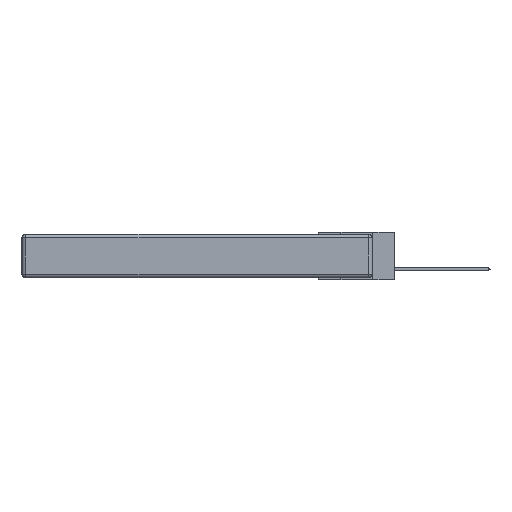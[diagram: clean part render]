
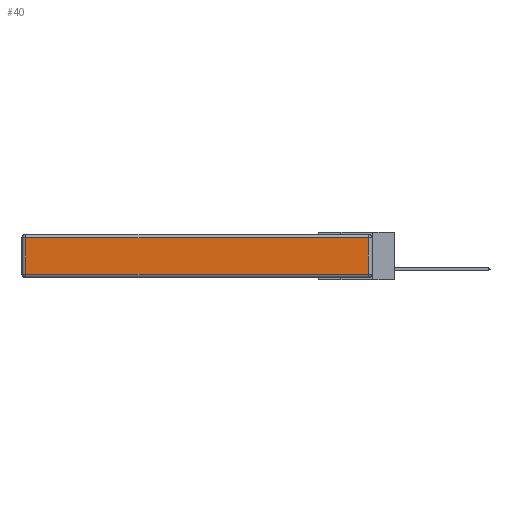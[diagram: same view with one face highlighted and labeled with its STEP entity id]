
A CAD part, left-side view. The second image highlights one B-rep face of the part: STEP entity #40.
In plain terms, the highlighted planar face has unit normal (-1, 0, 0).
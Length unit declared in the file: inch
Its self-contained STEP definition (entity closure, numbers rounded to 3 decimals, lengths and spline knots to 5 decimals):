
#40 = ADVANCED_FACE ( 'NONE', ( #24130 ), #11914, .T. ) ;
#485 = LINE ( 'NONE', #15157, #26127 ) ;
#1071 = EDGE_CURVE ( 'NONE', #5950, #18818, #15418, .T. ) ;
#2519 = ORIENTED_EDGE ( 'NONE', *, *, #5761, .T. ) ;
#3754 = DIRECTION ( 'NONE',  ( -1., 0., 0. ) ) ;
#3831 = VECTOR ( 'NONE', #7269, 39.37008 ) ;
#4460 = DIRECTION ( 'NONE',  ( 0., 0., -1. ) ) ;
#4803 = LINE ( 'NONE', #22928, #15100 ) ;
#5084 = CARTESIAN_POINT ( 'NONE',  ( 0., 2.72, -0.313 ) ) ;
#5466 = CARTESIAN_POINT ( 'NONE',  ( 0., 0.03, -0.343 ) ) ;
#5761 = EDGE_CURVE ( 'NONE', #18818, #6465, #485, .T. ) ;
#5910 = DIRECTION ( 'NONE',  ( 0., 0., 1. ) ) ;
#5950 = VERTEX_POINT ( 'NONE', #21276 ) ;
#6465 = VERTEX_POINT ( 'NONE', #13262 ) ;
#7269 = DIRECTION ( 'NONE',  ( 0., 0., 1. ) ) ;
#8043 = CARTESIAN_POINT ( 'NONE',  ( 0., 0., -0.343 ) ) ;
#11120 = EDGE_CURVE ( 'NONE', #17158, #5950, #4803, .T. ) ;
#11696 = ORIENTED_EDGE ( 'NONE', *, *, #11120, .T. ) ;
#11914 = PLANE ( 'NONE',  #11932 ) ;
#11932 = AXIS2_PLACEMENT_3D ( 'NONE', #8043, #3754, #5910 ) ;
#12120 = ORIENTED_EDGE ( 'NONE', *, *, #1071, .T. ) ;
#12388 = VECTOR ( 'NONE', #4460, 39.37008 ) ;
#12735 = EDGE_CURVE ( 'NONE', #6465, #17158, #19508, .T. ) ;
#13262 = CARTESIAN_POINT ( 'NONE',  ( 0., 2.72, -0.03 ) ) ;
#14337 = DIRECTION ( 'NONE',  ( 0., -1., 0. ) ) ;
#14644 = CARTESIAN_POINT ( 'NONE',  ( 0., 2.72, -0.343 ) ) ;
#15100 = VECTOR ( 'NONE', #14337, 39.37008 ) ;
#15157 = CARTESIAN_POINT ( 'NONE',  ( 0., 2.75, -0.03 ) ) ;
#15418 = LINE ( 'NONE', #5466, #3831 ) ;
#16150 = ORIENTED_EDGE ( 'NONE', *, *, #12735, .T. ) ;
#16777 = CARTESIAN_POINT ( 'NONE',  ( 0., 0.03, -0.03 ) ) ;
#17158 = VERTEX_POINT ( 'NONE', #5084 ) ;
#18818 = VERTEX_POINT ( 'NONE', #16777 ) ;
#19508 = LINE ( 'NONE', #14644, #12388 ) ;
#21191 = DIRECTION ( 'NONE',  ( 0., 1., 0. ) ) ;
#21276 = CARTESIAN_POINT ( 'NONE',  ( 0., 0.03, -0.313 ) ) ;
#22928 = CARTESIAN_POINT ( 'NONE',  ( 0., 0., -0.313 ) ) ;
#24130 = FACE_OUTER_BOUND ( 'NONE', #24866, .T. ) ;
#24866 = EDGE_LOOP ( 'NONE', ( #11696, #12120, #2519, #16150 ) ) ;
#26127 = VECTOR ( 'NONE', #21191, 39.37008 ) ;
